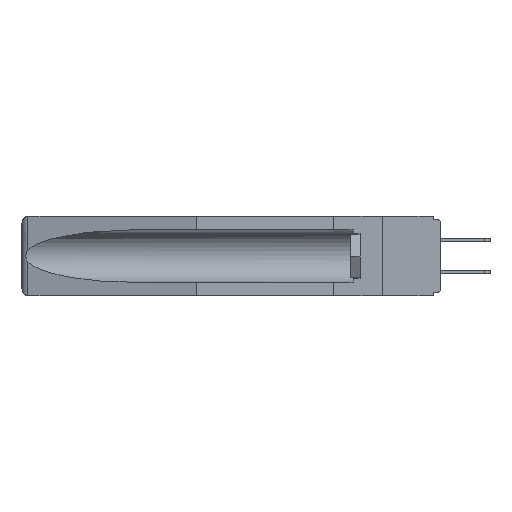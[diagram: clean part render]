
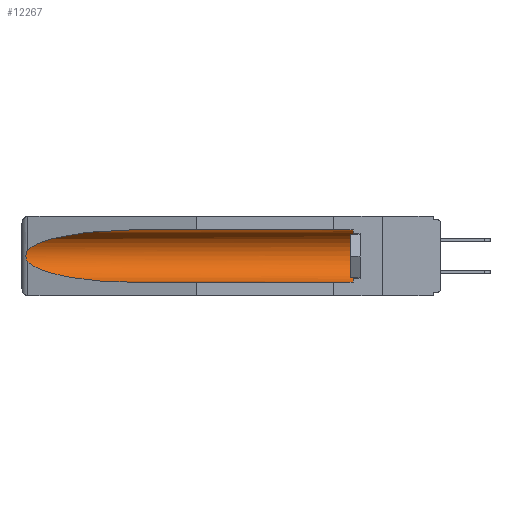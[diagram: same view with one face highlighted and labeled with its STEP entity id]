
A CAD part, left-side view. The second image highlights one B-rep face of the part: STEP entity #12267.
In plain terms, the highlighted cylindrical face has radius 2.857 mm (diameter 5.715 mm), a partial arc.
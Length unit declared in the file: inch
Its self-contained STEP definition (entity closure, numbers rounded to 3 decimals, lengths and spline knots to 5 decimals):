
#23 = CARTESIAN_POINT ( 'NONE',  ( 0.26654, 1.53092, -0.15636 ) ) ;
#1024 = VERTEX_POINT ( 'NONE', #2832 ) ;
#1136 = CARTESIAN_POINT ( 'NONE',  ( 0.26537, 1.52718, -0.14972 ) ) ;
#1336 = CARTESIAN_POINT ( 'NONE',  ( 0.25451, 1.48313, -0.24835 ) ) ;
#1631 = CARTESIAN_POINT ( 'NONE',  ( 0.155, 0.126, -0.284 ) ) ;
#1780 = CARTESIAN_POINT ( 'NONE',  ( 0.26597, 1.5296, -0.19026 ) ) ;
#2832 = CARTESIAN_POINT ( 'NONE',  ( 0.26537, 1.52718, -0.19328 ) ) ;
#3245 = CARTESIAN_POINT ( 'NONE',  ( 0.155, -0.30754, -0.284 ) ) ;
#3445 = ORIENTED_EDGE ( 'NONE', *, *, #20427, .F. ) ;
#3629 = CARTESIAN_POINT ( 'NONE',  ( 0.26597, 1.52961, -0.15275 ) ) ;
#4307 =( BOUNDED_CURVE ( )  B_SPLINE_CURVE ( 3, ( #18904, #1336, #6393, #9993 ),
 .UNSPECIFIED., .F., .F. ) 
 B_SPLINE_CURVE_WITH_KNOTS ( ( 4, 4 ),
 ( 0.1948, 1.5708 ),
 .UNSPECIFIED. ) 
 CURVE ( )  GEOMETRIC_REPRESENTATION_ITEM ( )  RATIONAL_B_SPLINE_CURVE ( ( 1., 0.848, 0.848, 1. ) ) 
 REPRESENTATION_ITEM ( '' )  );
#4864 = EDGE_LOOP ( 'NONE', ( #19902, #9729, #22767, #3445, #6920, #11244 ) ) ;
#5217 = CARTESIAN_POINT ( 'NONE',  ( 0.2675, 1.53308, -0.16763 ) ) ;
#5408 = DIRECTION ( 'NONE',  ( 0., 0., 1. ) ) ;
#5742 = CARTESIAN_POINT ( 'NONE',  ( 0.25451, 1.48313, -0.09465 ) ) ;
#5864 = LINE ( 'NONE', #3245, #17138 ) ;
#6393 = CARTESIAN_POINT ( 'NONE',  ( 0.21114, 1.30732, -0.284 ) ) ;
#6551 = CARTESIAN_POINT ( 'NONE',  ( 0.155, -0.30754, -0.059 ) ) ;
#6920 = ORIENTED_EDGE ( 'NONE', *, *, #20072, .T. ) ;
#7048 = CARTESIAN_POINT ( 'NONE',  ( 0.155, 0.126, -0.059 ) ) ;
#7069 = CARTESIAN_POINT ( 'NONE',  ( 0.2673, 1.53269, -0.17917 ) ) ;
#7996 = LINE ( 'NONE', #6551, #10755 ) ;
#8670 = CARTESIAN_POINT ( 'NONE',  ( 0.26655, 1.53094, -0.18657 ) ) ;
#8696 = DIRECTION ( 'NONE',  ( 0., 1., 0. ) ) ;
#8987 = FACE_OUTER_BOUND ( 'NONE', #4864, .T. ) ;
#9179 = DIRECTION ( 'NONE',  ( 0., -1., 0. ) ) ;
#9729 = ORIENTED_EDGE ( 'NONE', *, *, #18149, .T. ) ;
#9993 = CARTESIAN_POINT ( 'NONE',  ( 0.155, 1.07973, -0.284 ) ) ;
#10470 = AXIS2_PLACEMENT_3D ( 'NONE', #21576, #9179, #21951 ) ;
#10755 = VECTOR ( 'NONE', #15417, 39.37008 ) ;
#11244 = ORIENTED_EDGE ( 'NONE', *, *, #15389, .T. ) ;
#11717 = EDGE_CURVE ( 'NONE', #17311, #16236, #14173, .T. ) ;
#12019 = CYLINDRICAL_SURFACE ( 'NONE', #14222, 0.1125 ) ;
#12267 = ADVANCED_FACE ( 'NONE', ( #8987 ), #12019, .F. ) ;
#13565 = VERTEX_POINT ( 'NONE', #22687 ) ;
#14157 = CARTESIAN_POINT ( 'NONE',  ( 0.26537, 1.52718, -0.14972 ) ) ;
#14173 =( BOUNDED_CURVE ( )  B_SPLINE_CURVE ( 3, ( #16336, #14515, #5742, #18072 ),
 .UNSPECIFIED., .F., .F. ) 
 B_SPLINE_CURVE_WITH_KNOTS ( ( 4, 4 ),
 ( 4.71239, 6.08839 ),
 .UNSPECIFIED. ) 
 CURVE ( )  GEOMETRIC_REPRESENTATION_ITEM ( )  RATIONAL_B_SPLINE_CURVE ( ( 1., 0.848, 0.848, 1. ) ) 
 REPRESENTATION_ITEM ( '' )  );
#14222 = AXIS2_PLACEMENT_3D ( 'NONE', #21178, #8696, #5408 ) ;
#14515 = CARTESIAN_POINT ( 'NONE',  ( 0.21114, 1.30732, -0.059 ) ) ;
#14778 = VERTEX_POINT ( 'NONE', #1631 ) ;
#14985 = CIRCLE ( 'NONE', #10470, 0.1125 ) ;
#15389 = EDGE_CURVE ( 'NONE', #18747, #17311, #7996, .T. ) ;
#15417 = DIRECTION ( 'NONE',  ( 0., 1., 0. ) ) ;
#15563 = DIRECTION ( 'NONE',  ( 0., 1., 0. ) ) ;
#15841 = CARTESIAN_POINT ( 'NONE',  ( 0.2675, 1.53308, -0.17534 ) ) ;
#16236 = VERTEX_POINT ( 'NONE', #1136 ) ;
#16336 = CARTESIAN_POINT ( 'NONE',  ( 0.155, 1.07973, -0.059 ) ) ;
#16551 = B_SPLINE_CURVE_WITH_KNOTS ( 'NONE', 3,
 ( #14157, #3629, #23, #22745, #5217, #15841, #7069, #8670, #1780, #17567 ),
 .UNSPECIFIED., .F., .F.,
 ( 4, 2, 2, 2, 4 ),
 ( 0., 0.00029, 0.00058, 0.00087, 0.00117 ),
 .UNSPECIFIED. ) ;
#17138 = VECTOR ( 'NONE', #15563, 39.37008 ) ;
#17311 = VERTEX_POINT ( 'NONE', #18768 ) ;
#17567 = CARTESIAN_POINT ( 'NONE',  ( 0.26537, 1.52718, -0.19328 ) ) ;
#18072 = CARTESIAN_POINT ( 'NONE',  ( 0.26537, 1.52718, -0.14972 ) ) ;
#18149 = EDGE_CURVE ( 'NONE', #16236, #1024, #16551, .T. ) ;
#18747 = VERTEX_POINT ( 'NONE', #7048 ) ;
#18768 = CARTESIAN_POINT ( 'NONE',  ( 0.155, 1.07973, -0.059 ) ) ;
#18904 = CARTESIAN_POINT ( 'NONE',  ( 0.26537, 1.52718, -0.19328 ) ) ;
#19902 = ORIENTED_EDGE ( 'NONE', *, *, #11717, .T. ) ;
#20072 = EDGE_CURVE ( 'NONE', #14778, #18747, #14985, .T. ) ;
#20427 = EDGE_CURVE ( 'NONE', #14778, #13565, #5864, .T. ) ;
#21178 = CARTESIAN_POINT ( 'NONE',  ( 0.155, -0.30754, -0.1715 ) ) ;
#21576 = CARTESIAN_POINT ( 'NONE',  ( 0.155, 0.126, -0.1715 ) ) ;
#21951 = DIRECTION ( 'NONE',  ( 0., 0., 1. ) ) ;
#22645 = EDGE_CURVE ( 'NONE', #1024, #13565, #4307, .T. ) ;
#22687 = CARTESIAN_POINT ( 'NONE',  ( 0.155, 1.07973, -0.284 ) ) ;
#22745 = CARTESIAN_POINT ( 'NONE',  ( 0.2673, 1.5327, -0.16383 ) ) ;
#22767 = ORIENTED_EDGE ( 'NONE', *, *, #22645, .T. ) ;
